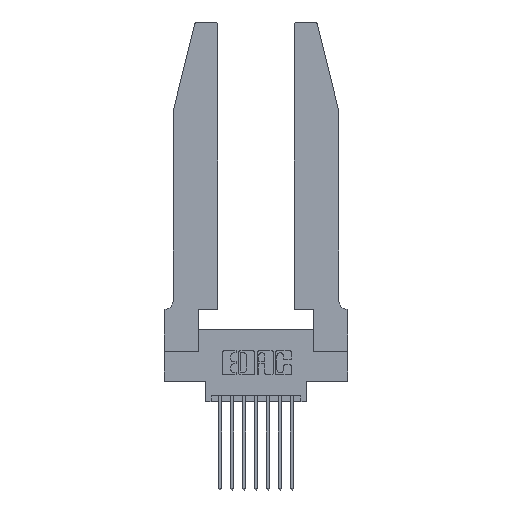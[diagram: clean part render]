
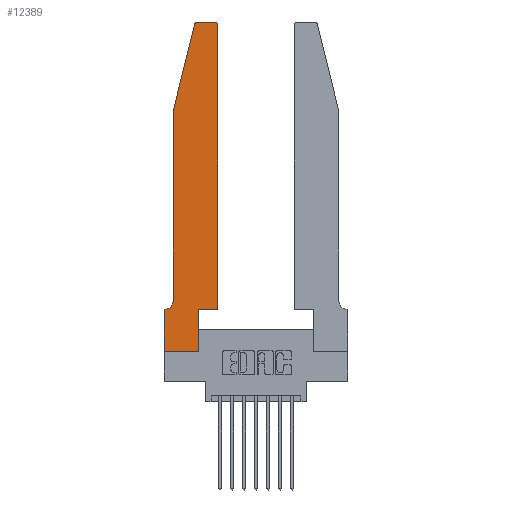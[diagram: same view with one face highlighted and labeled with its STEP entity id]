
A CAD part, top view. The second image highlights one B-rep face of the part: STEP entity #12389.
In plain terms, the highlighted planar face has unit normal (0, 0, 1).
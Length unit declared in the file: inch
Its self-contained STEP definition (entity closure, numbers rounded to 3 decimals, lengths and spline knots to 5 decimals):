
#16 = CARTESIAN_POINT ( 'NONE',  ( 0.2605, 2.75, 0.37 ) ) ;
#22 = ORIENTED_EDGE ( 'NONE', *, *, #10187, .T. ) ;
#160 = DIRECTION ( 'NONE',  ( 0., 1., 0. ) ) ;
#416 = LINE ( 'NONE', #2567, #10148 ) ;
#483 = CARTESIAN_POINT ( 'NONE',  ( 0.284, 2.75, 0.37 ) ) ;
#650 = CARTESIAN_POINT ( 'NONE',  ( 0.284, 2.72, 0.37 ) ) ;
#672 = CARTESIAN_POINT ( 'NONE',  ( 0.0755, 0.35, 0.37 ) ) ;
#835 = VERTEX_POINT ( 'NONE', #5781 ) ;
#922 = CARTESIAN_POINT ( 'NONE',  ( 0.4505, 0.35, 0.37 ) ) ;
#1041 = ORIENTED_EDGE ( 'NONE', *, *, #6873, .T. ) ;
#1098 = CARTESIAN_POINT ( 'NONE',  ( 0., 0., 0.37 ) ) ;
#1294 = DIRECTION ( 'NONE',  ( 0., 0., -1. ) ) ;
#1407 = VECTOR ( 'NONE', #2966, 39.37008 ) ;
#1506 = VERTEX_POINT ( 'NONE', #4553 ) ;
#1715 = VERTEX_POINT ( 'NONE', #13216 ) ;
#1843 = DIRECTION ( 'NONE',  ( 1., 0., 0. ) ) ;
#1860 = EDGE_CURVE ( 'NONE', #2170, #6382, #9360, .T. ) ;
#1942 = ORIENTED_EDGE ( 'NONE', *, *, #3995, .T. ) ;
#2079 = DIRECTION ( 'NONE',  ( 1., 0., 0. ) ) ;
#2170 = VERTEX_POINT ( 'NONE', #12822 ) ;
#2287 = FACE_OUTER_BOUND ( 'NONE', #14692, .T. ) ;
#2288 = CARTESIAN_POINT ( 'NONE',  ( 0.25487, 2.72718, 0.37 ) ) ;
#2446 = EDGE_CURVE ( 'NONE', #6382, #14536, #4736, .T. ) ;
#2567 = CARTESIAN_POINT ( 'NONE',  ( 0.4505, 0.35, 0.37 ) ) ;
#2768 = LINE ( 'NONE', #1098, #14425 ) ;
#2966 = DIRECTION ( 'NONE',  ( 1., 0., 0. ) ) ;
#3641 = VECTOR ( 'NONE', #8895, 39.37008 ) ;
#3726 = DIRECTION ( 'NONE',  ( 0., 1., 0. ) ) ;
#3980 = ORIENTED_EDGE ( 'NONE', *, *, #1860, .T. ) ;
#3995 = EDGE_CURVE ( 'NONE', #15102, #7776, #10029, .T. ) ;
#4553 = CARTESIAN_POINT ( 'NONE',  ( 0., 0., 0.37 ) ) ;
#4736 = CIRCLE ( 'NONE', #10412, 0.03 ) ;
#4888 = LINE ( 'NONE', #5248, #1407 ) ;
#5132 = AXIS2_PLACEMENT_3D ( 'NONE', #8328, #1294, #9503 ) ;
#5248 = CARTESIAN_POINT ( 'NONE',  ( 0., 0., 0.37 ) ) ;
#5485 = EDGE_CURVE ( 'NONE', #11905, #13949, #6898, .T. ) ;
#5606 = EDGE_CURVE ( 'NONE', #1715, #2170, #10869, .T. ) ;
#5781 = CARTESIAN_POINT ( 'NONE',  ( 0.0755, 2., 0.37 ) ) ;
#5860 = VECTOR ( 'NONE', #10843, 39.37008 ) ;
#5956 = ORIENTED_EDGE ( 'NONE', *, *, #6229, .T. ) ;
#6009 = DIRECTION ( 'NONE',  ( 0., -1., 0. ) ) ;
#6209 = CARTESIAN_POINT ( 'NONE',  ( 0.4205, 2.72, 0.37 ) ) ;
#6229 = EDGE_CURVE ( 'NONE', #7776, #1715, #416, .T. ) ;
#6382 = VERTEX_POINT ( 'NONE', #483 ) ;
#6605 = CARTESIAN_POINT ( 'NONE',  ( 0.0055, 0.35, 0.37 ) ) ;
#6873 = EDGE_CURVE ( 'NONE', #12493, #15102, #7969, .T. ) ;
#6898 = CIRCLE ( 'NONE', #5132, 0.07 ) ;
#6989 = ORIENTED_EDGE ( 'NONE', *, *, #5485, .T. ) ;
#7307 = VECTOR ( 'NONE', #8321, 39.37008 ) ;
#7312 = ORIENTED_EDGE ( 'NONE', *, *, #2446, .T. ) ;
#7327 = EDGE_CURVE ( 'NONE', #835, #11905, #9041, .T. ) ;
#7401 = DIRECTION ( 'NONE',  ( 1., 0., 0. ) ) ;
#7776 = VERTEX_POINT ( 'NONE', #922 ) ;
#7783 = ORIENTED_EDGE ( 'NONE', *, *, #8935, .T. ) ;
#7932 = PLANE ( 'NONE',  #8166 ) ;
#7969 = LINE ( 'NONE', #14148, #13735 ) ;
#8132 = CARTESIAN_POINT ( 'NONE',  ( 0.2865, 0., 0.37 ) ) ;
#8166 = AXIS2_PLACEMENT_3D ( 'NONE', #10147, #9102, #2079 ) ;
#8321 = DIRECTION ( 'NONE',  ( 1., 0., 0. ) ) ;
#8328 = CARTESIAN_POINT ( 'NONE',  ( 0.0055, 0.42, 0.37 ) ) ;
#8875 = DIRECTION ( 'NONE',  ( 0., 0., 1. ) ) ;
#8895 = DIRECTION ( 'NONE',  ( -1., 0., 0. ) ) ;
#8935 = EDGE_CURVE ( 'NONE', #14536, #835, #15124, .T. ) ;
#8994 = VECTOR ( 'NONE', #14369, 39.37008 ) ;
#9041 = LINE ( 'NONE', #12938, #14092 ) ;
#9102 = DIRECTION ( 'NONE',  ( 0., 0., 1. ) ) ;
#9128 = EDGE_CURVE ( 'NONE', #13949, #10210, #12178, .T. ) ;
#9360 = LINE ( 'NONE', #16, #8994 ) ;
#9503 = DIRECTION ( 'NONE',  ( -1., 0., 0. ) ) ;
#9841 = AXIS2_PLACEMENT_3D ( 'NONE', #6209, #14323, #7401 ) ;
#10029 = LINE ( 'NONE', #14080, #7307 ) ;
#10147 = CARTESIAN_POINT ( 'NONE',  ( 0., 0.35, 0.37 ) ) ;
#10148 = VECTOR ( 'NONE', #3726, 39.37008 ) ;
#10187 = EDGE_CURVE ( 'NONE', #1506, #12493, #4888, .T. ) ;
#10210 = VERTEX_POINT ( 'NONE', #14609 ) ;
#10363 = ORIENTED_EDGE ( 'NONE', *, *, #9128, .T. ) ;
#10412 = AXIS2_PLACEMENT_3D ( 'NONE', #650, #8875, #1843 ) ;
#10612 = ORIENTED_EDGE ( 'NONE', *, *, #5606, .T. ) ;
#10833 = ORIENTED_EDGE ( 'NONE', *, *, #14071, .T. ) ;
#10843 = DIRECTION ( 'NONE',  ( -0.239, -0.971, 0. ) ) ;
#10869 = CIRCLE ( 'NONE', #9841, 0.03 ) ;
#11905 = VERTEX_POINT ( 'NONE', #12693 ) ;
#11975 = CARTESIAN_POINT ( 'NONE',  ( 0.0755, 2., 0.37 ) ) ;
#12178 = LINE ( 'NONE', #672, #3641 ) ;
#12377 = ORIENTED_EDGE ( 'NONE', *, *, #7327, .T. ) ;
#12389 = ADVANCED_FACE ( 'NONE', ( #2287 ), #7932, .T. ) ;
#12493 = VERTEX_POINT ( 'NONE', #8132 ) ;
#12693 = CARTESIAN_POINT ( 'NONE',  ( 0.0755, 0.42, 0.37 ) ) ;
#12745 = DIRECTION ( 'NONE',  ( 0., -1., 0. ) ) ;
#12822 = CARTESIAN_POINT ( 'NONE',  ( 0.4205, 2.75, 0.37 ) ) ;
#12938 = CARTESIAN_POINT ( 'NONE',  ( 0.0755, 2., 0.37 ) ) ;
#13216 = CARTESIAN_POINT ( 'NONE',  ( 0.4505, 2.72, 0.37 ) ) ;
#13735 = VECTOR ( 'NONE', #160, 39.37008 ) ;
#13949 = VERTEX_POINT ( 'NONE', #6605 ) ;
#14071 = EDGE_CURVE ( 'NONE', #10210, #1506, #2768, .T. ) ;
#14080 = CARTESIAN_POINT ( 'NONE',  ( 0.4505, 0.35, 0.37 ) ) ;
#14092 = VECTOR ( 'NONE', #6009, 39.37008 ) ;
#14148 = CARTESIAN_POINT ( 'NONE',  ( 0.2865, 0.35, 0.37 ) ) ;
#14323 = DIRECTION ( 'NONE',  ( 0., 0., 1. ) ) ;
#14369 = DIRECTION ( 'NONE',  ( -1., 0., 0. ) ) ;
#14425 = VECTOR ( 'NONE', #12745, 39.37008 ) ;
#14536 = VERTEX_POINT ( 'NONE', #2288 ) ;
#14609 = CARTESIAN_POINT ( 'NONE',  ( 0., 0.35, 0.37 ) ) ;
#14692 = EDGE_LOOP ( 'NONE', ( #3980, #7312, #7783, #12377, #6989, #10363, #10833, #22, #1041, #1942, #5956, #10612 ) ) ;
#14993 = CARTESIAN_POINT ( 'NONE',  ( 0.2865, 0.35, 0.37 ) ) ;
#15102 = VERTEX_POINT ( 'NONE', #14993 ) ;
#15124 = LINE ( 'NONE', #11975, #5860 ) ;
